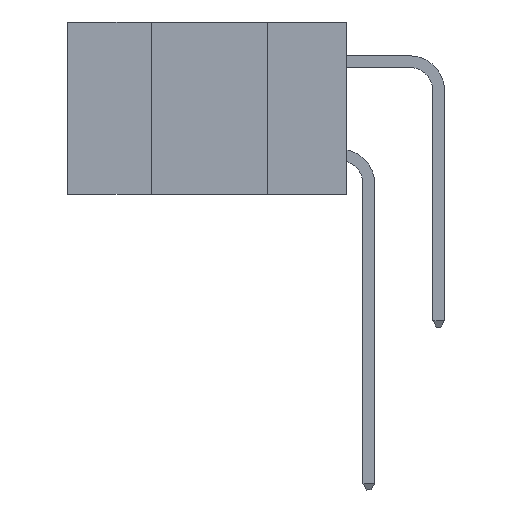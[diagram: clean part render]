
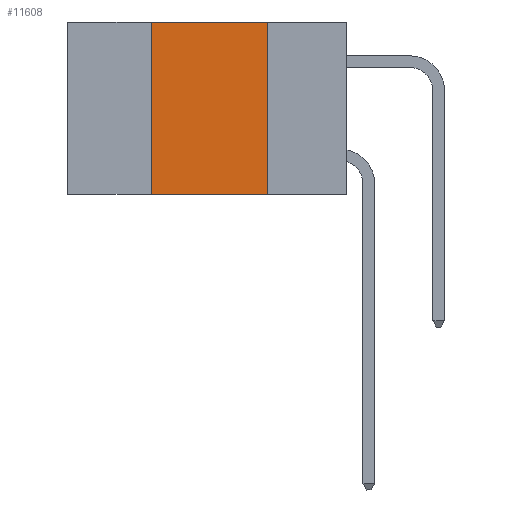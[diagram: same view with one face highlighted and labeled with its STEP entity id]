
A CAD part, left-side view. The second image highlights one B-rep face of the part: STEP entity #11608.
In plain terms, the highlighted planar face has unit normal (-1, 0, 0).
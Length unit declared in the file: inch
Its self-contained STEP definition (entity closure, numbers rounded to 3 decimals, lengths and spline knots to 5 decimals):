
#188 = ORIENTED_EDGE ( 'NONE', *, *, #4394, .T. ) ;
#881 = VECTOR ( 'NONE', #10680, 39.37008 ) ;
#1111 = VECTOR ( 'NONE', #11218, 39.37008 ) ;
#2494 = CARTESIAN_POINT ( 'NONE',  ( 0., 0.17, -0.37 ) ) ;
#2980 = VERTEX_POINT ( 'NONE', #2494 ) ;
#3379 = VECTOR ( 'NONE', #5215, 39.37008 ) ;
#3599 = AXIS2_PLACEMENT_3D ( 'NONE', #5558, #9557, #8171 ) ;
#4394 = EDGE_CURVE ( 'NONE', #11489, #2980, #10671, .T. ) ;
#4554 = LINE ( 'NONE', #11481, #11214 ) ;
#5080 = FACE_OUTER_BOUND ( 'NONE', #9277, .T. ) ;
#5215 = DIRECTION ( 'NONE',  ( 0., 0., 1. ) ) ;
#5507 = EDGE_CURVE ( 'NONE', #11489, #9893, #15213, .T. ) ;
#5558 = CARTESIAN_POINT ( 'NONE',  ( 0., 0.6, 0. ) ) ;
#5644 = EDGE_CURVE ( 'NONE', #9893, #8978, #15641, .T. ) ;
#6952 = EDGE_CURVE ( 'NONE', #8978, #2980, #4554, .T. ) ;
#7092 = ORIENTED_EDGE ( 'NONE', *, *, #6952, .F. ) ;
#8171 = DIRECTION ( 'NONE',  ( 0., 0., -1. ) ) ;
#8937 = CARTESIAN_POINT ( 'NONE',  ( 0., 0.42, 0. ) ) ;
#8978 = VERTEX_POINT ( 'NONE', #14317 ) ;
#9277 = EDGE_LOOP ( 'NONE', ( #7092, #16254, #12154, #188 ) ) ;
#9345 = CARTESIAN_POINT ( 'NONE',  ( 0., 0.42, -0.37 ) ) ;
#9446 = PLANE ( 'NONE',  #3599 ) ;
#9557 = DIRECTION ( 'NONE',  ( 1., 0., 0. ) ) ;
#9893 = VERTEX_POINT ( 'NONE', #8937 ) ;
#10039 = DIRECTION ( 'NONE',  ( 0., 0., -1. ) ) ;
#10671 = LINE ( 'NONE', #13838, #1111 ) ;
#10680 = DIRECTION ( 'NONE',  ( 0., -1., 0. ) ) ;
#11214 = VECTOR ( 'NONE', #10039, 39.37008 ) ;
#11218 = DIRECTION ( 'NONE',  ( 0., -1., 0. ) ) ;
#11481 = CARTESIAN_POINT ( 'NONE',  ( 0., 0.17, 0. ) ) ;
#11489 = VERTEX_POINT ( 'NONE', #9345 ) ;
#11608 = ADVANCED_FACE ( 'NONE', ( #5080 ), #9446, .F. ) ;
#12154 = ORIENTED_EDGE ( 'NONE', *, *, #5507, .F. ) ;
#13838 = CARTESIAN_POINT ( 'NONE',  ( 0., 0.6, -0.37 ) ) ;
#14317 = CARTESIAN_POINT ( 'NONE',  ( 0., 0.17, 0. ) ) ;
#14664 = CARTESIAN_POINT ( 'NONE',  ( 0., 0.6, 0. ) ) ;
#15213 = LINE ( 'NONE', #15997, #3379 ) ;
#15641 = LINE ( 'NONE', #14664, #881 ) ;
#15997 = CARTESIAN_POINT ( 'NONE',  ( 0., 0.42, 0. ) ) ;
#16254 = ORIENTED_EDGE ( 'NONE', *, *, #5644, .F. ) ;
